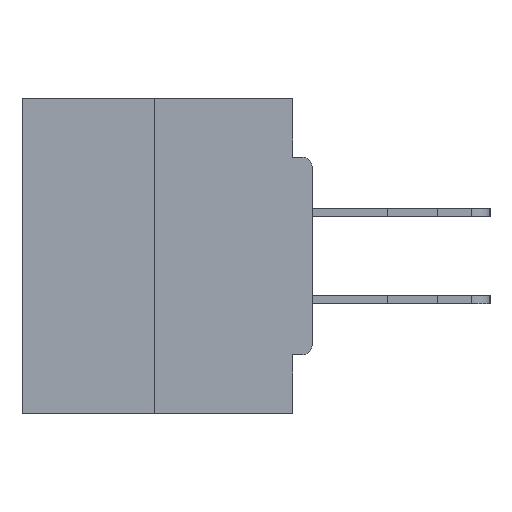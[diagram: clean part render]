
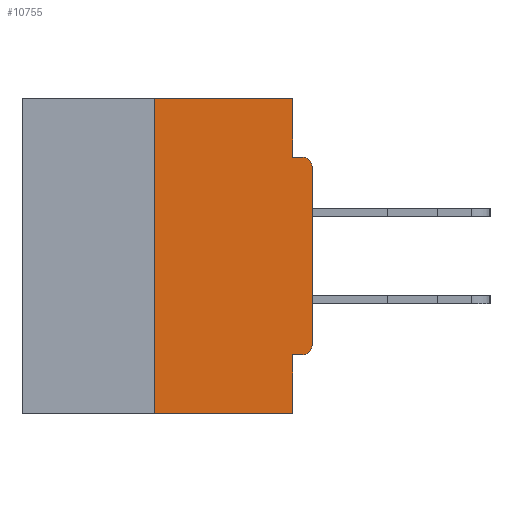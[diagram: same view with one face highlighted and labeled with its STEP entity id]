
A CAD part, left-side view. The second image highlights one B-rep face of the part: STEP entity #10755.
In plain terms, the highlighted planar face has unit normal (-1, 0, 0).
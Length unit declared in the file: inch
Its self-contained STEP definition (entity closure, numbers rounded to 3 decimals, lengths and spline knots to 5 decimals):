
#700 = VERTEX_POINT ( 'NONE', #17064 ) ;
#954 = VECTOR ( 'NONE', #19391, 39.37008 ) ;
#1150 = FACE_OUTER_BOUND ( 'NONE', #33064, .T. ) ;
#1375 = CARTESIAN_POINT ( 'NONE',  ( 0., 0.031, 0. ) ) ;
#1957 = ORIENTED_EDGE ( 'NONE', *, *, #33181, .F. ) ;
#2495 = CARTESIAN_POINT ( 'NONE',  ( 0., 0.031, -0.5 ) ) ;
#3177 = CARTESIAN_POINT ( 'NONE',  ( 0., 0.031, -0.0935 ) ) ;
#3363 = CARTESIAN_POINT ( 'NONE',  ( 0., 0., -0.4065 ) ) ;
#3375 = EDGE_CURVE ( 'NONE', #22738, #13594, #28421, .T. ) ;
#3480 = ORIENTED_EDGE ( 'NONE', *, *, #31019, .F. ) ;
#3498 = EDGE_CURVE ( 'NONE', #10458, #24117, #6058, .T. ) ;
#4395 = CARTESIAN_POINT ( 'NONE',  ( 0., 0.015, -0.1085 ) ) ;
#4888 = VERTEX_POINT ( 'NONE', #20773 ) ;
#4979 = CARTESIAN_POINT ( 'NONE',  ( 0., 0.46, 0. ) ) ;
#5093 = DIRECTION ( 'NONE',  ( 0., 0., -1. ) ) ;
#5554 = VECTOR ( 'NONE', #24602, 39.37008 ) ;
#5698 = CARTESIAN_POINT ( 'NONE',  ( 0., 0.25, -0.5 ) ) ;
#6058 = LINE ( 'NONE', #13938, #25552 ) ;
#6392 = DIRECTION ( 'NONE',  ( 0., -1., 0. ) ) ;
#6451 = AXIS2_PLACEMENT_3D ( 'NONE', #4979, #21239, #5093 ) ;
#6975 = DIRECTION ( 'NONE',  ( 0., 0., -1. ) ) ;
#7329 = ORIENTED_EDGE ( 'NONE', *, *, #28393, .T. ) ;
#7474 = CARTESIAN_POINT ( 'NONE',  ( 0., 0.015, -0.4065 ) ) ;
#8415 = ORIENTED_EDGE ( 'NONE', *, *, #19661, .F. ) ;
#8587 = ORIENTED_EDGE ( 'NONE', *, *, #3498, .F. ) ;
#8773 = VERTEX_POINT ( 'NONE', #5698 ) ;
#8915 = LINE ( 'NONE', #1375, #26725 ) ;
#9001 = EDGE_CURVE ( 'NONE', #700, #4888, #23255, .T. ) ;
#9829 = EDGE_CURVE ( 'NONE', #4888, #13594, #32785, .T. ) ;
#10089 = DIRECTION ( 'NONE',  ( 0., -1., 0. ) ) ;
#10263 = CARTESIAN_POINT ( 'NONE',  ( 0., 0.25, 0. ) ) ;
#10458 = VERTEX_POINT ( 'NONE', #10263 ) ;
#10755 = ADVANCED_FACE ( 'NONE', ( #1150 ), #26666, .F. ) ;
#10989 = CARTESIAN_POINT ( 'NONE',  ( 0., 0.015, -0.0935 ) ) ;
#11162 = VECTOR ( 'NONE', #19937, 39.37008 ) ;
#12371 = LINE ( 'NONE', #21166, #25257 ) ;
#12786 = CARTESIAN_POINT ( 'NONE',  ( 0., 0.015, -0.3915 ) ) ;
#12790 = ORIENTED_EDGE ( 'NONE', *, *, #9001, .T. ) ;
#13594 = VERTEX_POINT ( 'NONE', #10989 ) ;
#13938 = CARTESIAN_POINT ( 'NONE',  ( 0., 0.46, 0. ) ) ;
#14125 = ORIENTED_EDGE ( 'NONE', *, *, #21508, .T. ) ;
#14939 = DIRECTION ( 'NONE',  ( 0., 0., 1. ) ) ;
#15003 = ORIENTED_EDGE ( 'NONE', *, *, #34312, .F. ) ;
#16203 = ORIENTED_EDGE ( 'NONE', *, *, #9829, .T. ) ;
#16845 = CARTESIAN_POINT ( 'NONE',  ( 0., 0.031, -0.4065 ) ) ;
#17064 = CARTESIAN_POINT ( 'NONE',  ( 0., 0., -0.3915 ) ) ;
#19143 = CIRCLE ( 'NONE', #32024, 0.015 ) ;
#19391 = DIRECTION ( 'NONE',  ( 0., 1., 0. ) ) ;
#19661 = EDGE_CURVE ( 'NONE', #26640, #31957, #12371, .T. ) ;
#19937 = DIRECTION ( 'NONE',  ( 0., -1., 0. ) ) ;
#20206 = DIRECTION ( 'NONE',  ( 0., 0., -1. ) ) ;
#20773 = CARTESIAN_POINT ( 'NONE',  ( 0., 0., -0.1085 ) ) ;
#21166 = CARTESIAN_POINT ( 'NONE',  ( 0., 0.031, -0.5 ) ) ;
#21239 = DIRECTION ( 'NONE',  ( 1., 0., 0. ) ) ;
#21306 = CARTESIAN_POINT ( 'NONE',  ( 0., 0.031, 0. ) ) ;
#21508 = EDGE_CURVE ( 'NONE', #26944, #700, #19143, .T. ) ;
#21783 = ORIENTED_EDGE ( 'NONE', *, *, #3375, .F. ) ;
#22433 = VECTOR ( 'NONE', #14939, 39.37008 ) ;
#22680 = VECTOR ( 'NONE', #10089, 39.37008 ) ;
#22738 = VERTEX_POINT ( 'NONE', #3177 ) ;
#23255 = LINE ( 'NONE', #33395, #22433 ) ;
#23335 = CARTESIAN_POINT ( 'NONE',  ( 0., 0., -0.0935 ) ) ;
#23478 = DIRECTION ( 'NONE',  ( 0., 0., -1. ) ) ;
#23811 = LINE ( 'NONE', #3363, #954 ) ;
#24117 = VERTEX_POINT ( 'NONE', #21306 ) ;
#24602 = DIRECTION ( 'NONE',  ( 0., 0., 1. ) ) ;
#25257 = VECTOR ( 'NONE', #29017, 39.37008 ) ;
#25552 = VECTOR ( 'NONE', #6392, 39.37008 ) ;
#25636 = DIRECTION ( 'NONE',  ( -1., 0., 0. ) ) ;
#25677 = LINE ( 'NONE', #28001, #11162 ) ;
#26640 = VERTEX_POINT ( 'NONE', #16845 ) ;
#26666 = PLANE ( 'NONE',  #6451 ) ;
#26725 = VECTOR ( 'NONE', #20206, 39.37008 ) ;
#26944 = VERTEX_POINT ( 'NONE', #7474 ) ;
#27947 = LINE ( 'NONE', #30006, #5554 ) ;
#28001 = CARTESIAN_POINT ( 'NONE',  ( 0., 0.46, -0.5 ) ) ;
#28393 = EDGE_CURVE ( 'NONE', #8773, #31957, #25677, .T. ) ;
#28421 = LINE ( 'NONE', #23335, #22680 ) ;
#29017 = DIRECTION ( 'NONE',  ( 0., 0., -1. ) ) ;
#30006 = CARTESIAN_POINT ( 'NONE',  ( 0., 0.25, 0. ) ) ;
#31019 = EDGE_CURVE ( 'NONE', #8773, #10458, #27947, .T. ) ;
#31520 = AXIS2_PLACEMENT_3D ( 'NONE', #4395, #25636, #6975 ) ;
#31957 = VERTEX_POINT ( 'NONE', #2495 ) ;
#32024 = AXIS2_PLACEMENT_3D ( 'NONE', #12786, #33790, #23478 ) ;
#32785 = CIRCLE ( 'NONE', #31520, 0.015 ) ;
#33064 = EDGE_LOOP ( 'NONE', ( #8587, #3480, #7329, #8415, #15003, #14125, #12790, #16203, #21783, #1957 ) ) ;
#33181 = EDGE_CURVE ( 'NONE', #24117, #22738, #8915, .T. ) ;
#33395 = CARTESIAN_POINT ( 'NONE',  ( 0., 0., 0. ) ) ;
#33790 = DIRECTION ( 'NONE',  ( -1., 0., 0. ) ) ;
#34312 = EDGE_CURVE ( 'NONE', #26944, #26640, #23811, .T. ) ;
